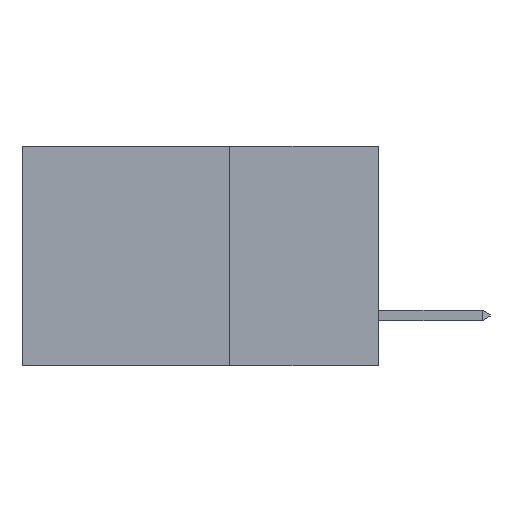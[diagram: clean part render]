
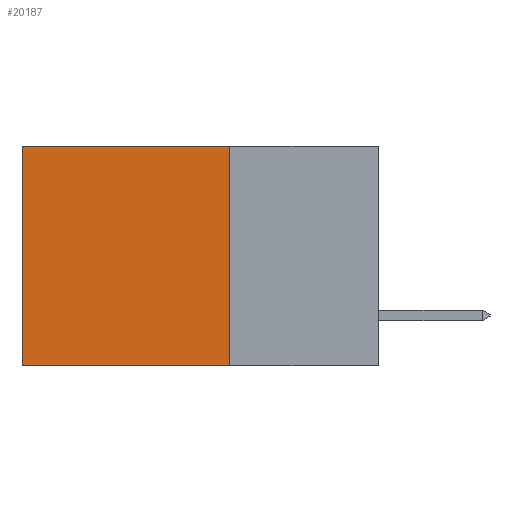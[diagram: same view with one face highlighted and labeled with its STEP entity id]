
A CAD part, left-side view. The second image highlights one B-rep face of the part: STEP entity #20187.
In plain terms, the highlighted planar face has unit normal (-1, 0, 0).
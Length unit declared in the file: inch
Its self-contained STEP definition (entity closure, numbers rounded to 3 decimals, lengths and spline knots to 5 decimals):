
#1222 = CARTESIAN_POINT ( 'NONE',  ( 0.2615, 0.25, -0.37 ) ) ;
#1884 = ORIENTED_EDGE ( 'NONE', *, *, #23417, .F. ) ;
#2420 = CARTESIAN_POINT ( 'NONE',  ( 0.2615, 0.25, 0. ) ) ;
#3263 = ORIENTED_EDGE ( 'NONE', *, *, #14115, .T. ) ;
#4385 = EDGE_CURVE ( 'NONE', #10093, #7668, #5881, .T. ) ;
#4461 = DIRECTION ( 'NONE',  ( 0., 1., 0. ) ) ;
#5881 = LINE ( 'NONE', #25029, #9935 ) ;
#7130 = ORIENTED_EDGE ( 'NONE', *, *, #4385, .F. ) ;
#7184 = EDGE_LOOP ( 'NONE', ( #21185, #7130, #1884, #3263 ) ) ;
#7668 = VERTEX_POINT ( 'NONE', #15098 ) ;
#7843 = CARTESIAN_POINT ( 'NONE',  ( 0.2615, 0.6, 0. ) ) ;
#8027 = FACE_OUTER_BOUND ( 'NONE', #7184, .T. ) ;
#9900 = CARTESIAN_POINT ( 'NONE',  ( 0.2615, 0.6, -0.37 ) ) ;
#9935 = VECTOR ( 'NONE', #10292, 39.37008 ) ;
#10093 = VERTEX_POINT ( 'NONE', #1222 ) ;
#10292 = DIRECTION ( 'NONE',  ( 0., 1., 0. ) ) ;
#11563 = CARTESIAN_POINT ( 'NONE',  ( 0.2615, 0.25, -0.37 ) ) ;
#12032 = DIRECTION ( 'NONE',  ( 0., 0., -1. ) ) ;
#12987 = VERTEX_POINT ( 'NONE', #7843 ) ;
#13524 = DIRECTION ( 'NONE',  ( 0., 0., -1. ) ) ;
#14115 = EDGE_CURVE ( 'NONE', #21259, #12987, #18592, .T. ) ;
#15029 = LINE ( 'NONE', #23653, #25328 ) ;
#15098 = CARTESIAN_POINT ( 'NONE',  ( 0.2615, 0.6, -0.37 ) ) ;
#18438 = CARTESIAN_POINT ( 'NONE',  ( 0.2615, 0.25, 0. ) ) ;
#18592 = LINE ( 'NONE', #2420, #22538 ) ;
#19342 = PLANE ( 'NONE',  #24832 ) ;
#19676 = DIRECTION ( 'NONE',  ( 0., 0., -1. ) ) ;
#20187 = ADVANCED_FACE ( 'NONE', ( #8027 ), #19342, .F. ) ;
#21185 = ORIENTED_EDGE ( 'NONE', *, *, #22256, .T. ) ;
#21259 = VERTEX_POINT ( 'NONE', #18438 ) ;
#21801 = VECTOR ( 'NONE', #19676, 39.37008 ) ;
#22256 = EDGE_CURVE ( 'NONE', #12987, #7668, #23002, .T. ) ;
#22538 = VECTOR ( 'NONE', #4461, 39.37008 ) ;
#23002 = LINE ( 'NONE', #9900, #21801 ) ;
#23417 = EDGE_CURVE ( 'NONE', #21259, #10093, #15029, .T. ) ;
#23653 = CARTESIAN_POINT ( 'NONE',  ( 0.2615, 0.25, -0.37 ) ) ;
#24832 = AXIS2_PLACEMENT_3D ( 'NONE', #11563, #25131, #13524 ) ;
#25029 = CARTESIAN_POINT ( 'NONE',  ( 0.2615, 0.25, -0.37 ) ) ;
#25131 = DIRECTION ( 'NONE',  ( 1., 0., 0. ) ) ;
#25328 = VECTOR ( 'NONE', #12032, 39.37008 ) ;
